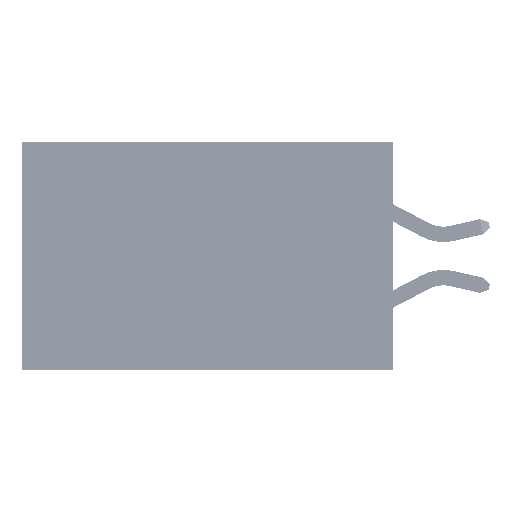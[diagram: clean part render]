
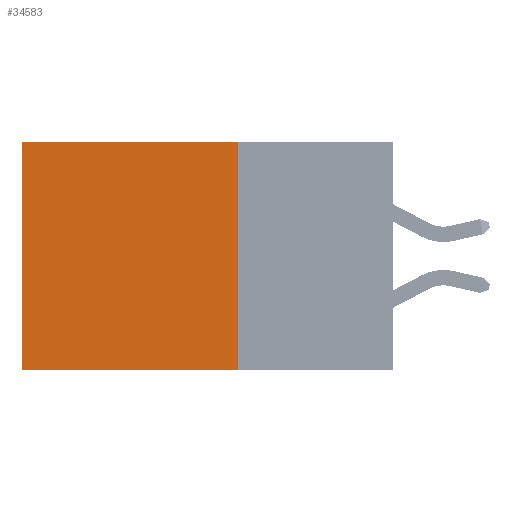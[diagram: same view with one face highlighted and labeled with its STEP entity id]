
A CAD part, left-side view. The second image highlights one B-rep face of the part: STEP entity #34583.
In plain terms, the highlighted planar face has unit normal (-1, 0, 0).
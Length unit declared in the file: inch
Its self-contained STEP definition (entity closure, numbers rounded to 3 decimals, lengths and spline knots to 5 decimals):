
#1493 = PLANE ( 'NONE',  #18995 ) ;
#2372 = LINE ( 'NONE', #23743, #25142 ) ;
#3937 = LINE ( 'NONE', #33616, #39609 ) ;
#7334 = ORIENTED_EDGE ( 'NONE', *, *, #31921, .F. ) ;
#8453 = CARTESIAN_POINT ( 'NONE',  ( 0.2875, 0.25, -0.37 ) ) ;
#10559 = LINE ( 'NONE', #19880, #17794 ) ;
#13334 = DIRECTION ( 'NONE',  ( 0., 1., 0. ) ) ;
#14508 = LINE ( 'NONE', #43565, #16751 ) ;
#15852 = DIRECTION ( 'NONE',  ( 0., 0., -1. ) ) ;
#16751 = VECTOR ( 'NONE', #43731, 39.37008 ) ;
#17758 = ORIENTED_EDGE ( 'NONE', *, *, #45067, .T. ) ;
#17794 = VECTOR ( 'NONE', #37806, 39.37008 ) ;
#17934 = VERTEX_POINT ( 'NONE', #29907 ) ;
#18995 = AXIS2_PLACEMENT_3D ( 'NONE', #19221, #44303, #30128 ) ;
#19221 = CARTESIAN_POINT ( 'NONE',  ( 0.2875, 0.25, 0. ) ) ;
#19880 = CARTESIAN_POINT ( 'NONE',  ( 0.2875, 0.6, 0. ) ) ;
#20134 = CARTESIAN_POINT ( 'NONE',  ( 0.2875, 0.6, 0. ) ) ;
#20151 = EDGE_CURVE ( 'NONE', #35670, #17934, #2372, .T. ) ;
#23743 = CARTESIAN_POINT ( 'NONE',  ( 0.2875, 0.25, -0.37 ) ) ;
#25142 = VECTOR ( 'NONE', #13334, 39.37008 ) ;
#25166 = VERTEX_POINT ( 'NONE', #20134 ) ;
#25248 = VERTEX_POINT ( 'NONE', #32149 ) ;
#29907 = CARTESIAN_POINT ( 'NONE',  ( 0.2875, 0.6, -0.37 ) ) ;
#30128 = DIRECTION ( 'NONE',  ( 0., 0., -1. ) ) ;
#31921 = EDGE_CURVE ( 'NONE', #25248, #35670, #3937, .T. ) ;
#32149 = CARTESIAN_POINT ( 'NONE',  ( 0.2875, 0.25, 0. ) ) ;
#33616 = CARTESIAN_POINT ( 'NONE',  ( 0.2875, 0.25, 0. ) ) ;
#33758 = ORIENTED_EDGE ( 'NONE', *, *, #33970, .T. ) ;
#33970 = EDGE_CURVE ( 'NONE', #25166, #17934, #10559, .T. ) ;
#34583 = ADVANCED_FACE ( 'NONE', ( #43979 ), #1493, .F. ) ;
#35670 = VERTEX_POINT ( 'NONE', #8453 ) ;
#37806 = DIRECTION ( 'NONE',  ( 0., 0., -1. ) ) ;
#39609 = VECTOR ( 'NONE', #15852, 39.37008 ) ;
#40590 = EDGE_LOOP ( 'NONE', ( #33758, #45385, #7334, #17758 ) ) ;
#43565 = CARTESIAN_POINT ( 'NONE',  ( 0.2875, 0.25, 0. ) ) ;
#43731 = DIRECTION ( 'NONE',  ( 0., 1., 0. ) ) ;
#43979 = FACE_OUTER_BOUND ( 'NONE', #40590, .T. ) ;
#44303 = DIRECTION ( 'NONE',  ( 1., 0., 0. ) ) ;
#45067 = EDGE_CURVE ( 'NONE', #25248, #25166, #14508, .T. ) ;
#45385 = ORIENTED_EDGE ( 'NONE', *, *, #20151, .F. ) ;
